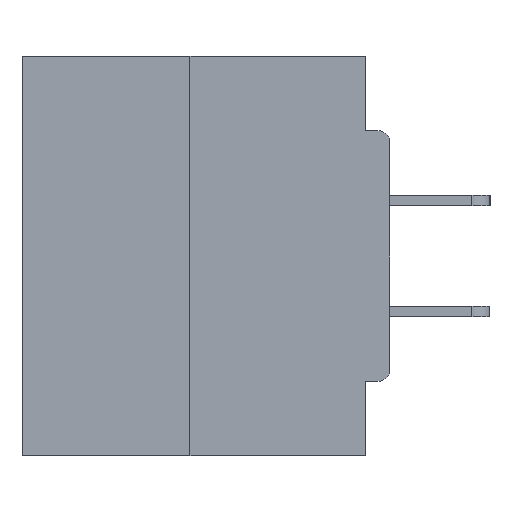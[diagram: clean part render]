
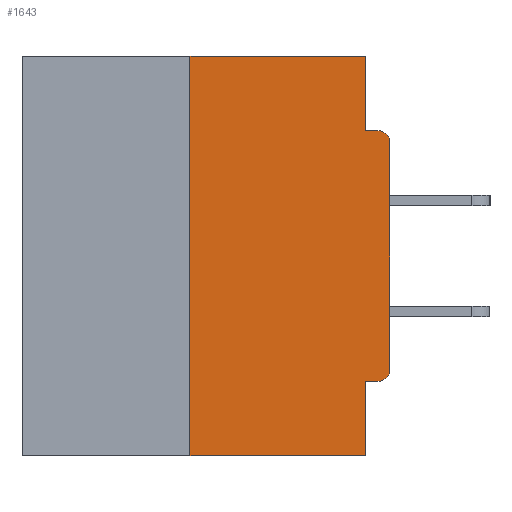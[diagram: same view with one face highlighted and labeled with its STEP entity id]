
A CAD part, left-side view. The second image highlights one B-rep face of the part: STEP entity #1643.
In plain terms, the highlighted planar face has unit normal (-1, 0, 0).
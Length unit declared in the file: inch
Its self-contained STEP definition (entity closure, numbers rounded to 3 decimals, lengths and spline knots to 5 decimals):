
#426 = EDGE_CURVE ( 'NONE', #15007, #32428, #3552, .T. ) ;
#1168 = VERTEX_POINT ( 'NONE', #11017 ) ;
#1373 = DIRECTION ( 'NONE',  ( -1., 0., 0. ) ) ;
#1518 = ORIENTED_EDGE ( 'NONE', *, *, #11115, .T. ) ;
#1625 = DIRECTION ( 'NONE',  ( 0., -1., 0. ) ) ;
#1643 = ADVANCED_FACE ( 'NONE', ( #10968 ), #23480, .F. ) ;
#1912 = VECTOR ( 'NONE', #2212, 39.37008 ) ;
#2177 = DIRECTION ( 'NONE',  ( 0., 0., -1. ) ) ;
#2212 = DIRECTION ( 'NONE',  ( 0., 0., -1. ) ) ;
#3349 = EDGE_LOOP ( 'NONE', ( #33163, #32352, #4244, #10885, #8279, #23006, #15114, #1518, #21735, #7559 ) ) ;
#3552 = LINE ( 'NONE', #21575, #23496 ) ;
#4244 = ORIENTED_EDGE ( 'NONE', *, *, #26829, .T. ) ;
#5197 = CARTESIAN_POINT ( 'NONE',  ( 0., 0.031, 0. ) ) ;
#5918 = LINE ( 'NONE', #31744, #19441 ) ;
#6201 = DIRECTION ( 'NONE',  ( 0., 0., -1. ) ) ;
#6227 = DIRECTION ( 'NONE',  ( 0., 0., -1. ) ) ;
#6773 = AXIS2_PLACEMENT_3D ( 'NONE', #18998, #13812, #6201 ) ;
#6791 = AXIS2_PLACEMENT_3D ( 'NONE', #8580, #1373, #6227 ) ;
#6827 = LINE ( 'NONE', #19303, #11557 ) ;
#7043 = EDGE_CURVE ( 'NONE', #21998, #25879, #22693, .T. ) ;
#7559 = ORIENTED_EDGE ( 'NONE', *, *, #16140, .F. ) ;
#8279 = ORIENTED_EDGE ( 'NONE', *, *, #7043, .F. ) ;
#8421 = DIRECTION ( 'NONE',  ( 0., 0., 1. ) ) ;
#8580 = CARTESIAN_POINT ( 'NONE',  ( 0., 0.015, -0.3915 ) ) ;
#8800 = VERTEX_POINT ( 'NONE', #30418 ) ;
#9622 = LINE ( 'NONE', #22606, #1912 ) ;
#10885 = ORIENTED_EDGE ( 'NONE', *, *, #16871, .F. ) ;
#10968 = FACE_OUTER_BOUND ( 'NONE', #3349, .T. ) ;
#11017 = CARTESIAN_POINT ( 'NONE',  ( 0., 0.015, -0.0935 ) ) ;
#11115 = EDGE_CURVE ( 'NONE', #32428, #1168, #12683, .T. ) ;
#11265 = DIRECTION ( 'NONE',  ( 0., -1., 0. ) ) ;
#11557 = VECTOR ( 'NONE', #1625, 39.37008 ) ;
#12683 = CIRCLE ( 'NONE', #6773, 0.015 ) ;
#12929 = LINE ( 'NONE', #5197, #29817 ) ;
#12984 = AXIS2_PLACEMENT_3D ( 'NONE', #21267, #15689, #25963 ) ;
#13492 = CARTESIAN_POINT ( 'NONE',  ( 0., 0., -0.1085 ) ) ;
#13694 = DIRECTION ( 'NONE',  ( 0., 0., 1. ) ) ;
#13812 = DIRECTION ( 'NONE',  ( -1., 0., 0. ) ) ;
#13869 = CARTESIAN_POINT ( 'NONE',  ( 0., 0., -0.0935 ) ) ;
#15007 = VERTEX_POINT ( 'NONE', #21420 ) ;
#15095 = DIRECTION ( 'NONE',  ( 0., 1., 0. ) ) ;
#15114 = ORIENTED_EDGE ( 'NONE', *, *, #426, .T. ) ;
#15403 = CIRCLE ( 'NONE', #6791, 0.015 ) ;
#15689 = DIRECTION ( 'NONE',  ( 1., 0., 0. ) ) ;
#15766 = CARTESIAN_POINT ( 'NONE',  ( 0., 0.031, -0.0935 ) ) ;
#16140 = EDGE_CURVE ( 'NONE', #8800, #19881, #12929, .T. ) ;
#16722 = EDGE_CURVE ( 'NONE', #19881, #1168, #29689, .T. ) ;
#16871 = EDGE_CURVE ( 'NONE', #25879, #31850, #9622, .T. ) ;
#18179 = VERTEX_POINT ( 'NONE', #20555 ) ;
#18998 = CARTESIAN_POINT ( 'NONE',  ( 0., 0.015, -0.1085 ) ) ;
#19303 = CARTESIAN_POINT ( 'NONE',  ( 0., 0.46, 0. ) ) ;
#19441 = VECTOR ( 'NONE', #13694, 39.37008 ) ;
#19881 = VERTEX_POINT ( 'NONE', #15766 ) ;
#20034 = EDGE_CURVE ( 'NONE', #32572, #8800, #6827, .T. ) ;
#20555 = CARTESIAN_POINT ( 'NONE',  ( 0., 0.25, -0.5 ) ) ;
#21267 = CARTESIAN_POINT ( 'NONE',  ( 0., 0.46, 0. ) ) ;
#21391 = VECTOR ( 'NONE', #11265, 39.37008 ) ;
#21420 = CARTESIAN_POINT ( 'NONE',  ( 0., 0., -0.3915 ) ) ;
#21575 = CARTESIAN_POINT ( 'NONE',  ( 0., 0., 0. ) ) ;
#21662 = EDGE_CURVE ( 'NONE', #21998, #15007, #15403, .T. ) ;
#21735 = ORIENTED_EDGE ( 'NONE', *, *, #16722, .F. ) ;
#21740 = CARTESIAN_POINT ( 'NONE',  ( 0., 0.25, 0. ) ) ;
#21998 = VERTEX_POINT ( 'NONE', #24410 ) ;
#22486 = CARTESIAN_POINT ( 'NONE',  ( 0., 0.031, -0.5 ) ) ;
#22606 = CARTESIAN_POINT ( 'NONE',  ( 0., 0.031, -0.5 ) ) ;
#22693 = LINE ( 'NONE', #30269, #28724 ) ;
#23006 = ORIENTED_EDGE ( 'NONE', *, *, #21662, .T. ) ;
#23480 = PLANE ( 'NONE',  #12984 ) ;
#23496 = VECTOR ( 'NONE', #8421, 39.37008 ) ;
#24311 = DIRECTION ( 'NONE',  ( 0., -1., 0. ) ) ;
#24410 = CARTESIAN_POINT ( 'NONE',  ( 0., 0.015, -0.4065 ) ) ;
#25879 = VERTEX_POINT ( 'NONE', #31251 ) ;
#25963 = DIRECTION ( 'NONE',  ( 0., 0., -1. ) ) ;
#26829 = EDGE_CURVE ( 'NONE', #18179, #31850, #28444, .T. ) ;
#28444 = LINE ( 'NONE', #28961, #21391 ) ;
#28724 = VECTOR ( 'NONE', #15095, 39.37008 ) ;
#28961 = CARTESIAN_POINT ( 'NONE',  ( 0., 0.46, -0.5 ) ) ;
#29347 = VECTOR ( 'NONE', #24311, 39.37008 ) ;
#29689 = LINE ( 'NONE', #13869, #29347 ) ;
#29817 = VECTOR ( 'NONE', #2177, 39.37008 ) ;
#30269 = CARTESIAN_POINT ( 'NONE',  ( 0., 0., -0.4065 ) ) ;
#30418 = CARTESIAN_POINT ( 'NONE',  ( 0., 0.031, 0. ) ) ;
#31112 = EDGE_CURVE ( 'NONE', #18179, #32572, #5918, .T. ) ;
#31251 = CARTESIAN_POINT ( 'NONE',  ( 0., 0.031, -0.4065 ) ) ;
#31744 = CARTESIAN_POINT ( 'NONE',  ( 0., 0.25, 0. ) ) ;
#31850 = VERTEX_POINT ( 'NONE', #22486 ) ;
#32352 = ORIENTED_EDGE ( 'NONE', *, *, #31112, .F. ) ;
#32428 = VERTEX_POINT ( 'NONE', #13492 ) ;
#32572 = VERTEX_POINT ( 'NONE', #21740 ) ;
#33163 = ORIENTED_EDGE ( 'NONE', *, *, #20034, .F. ) ;
